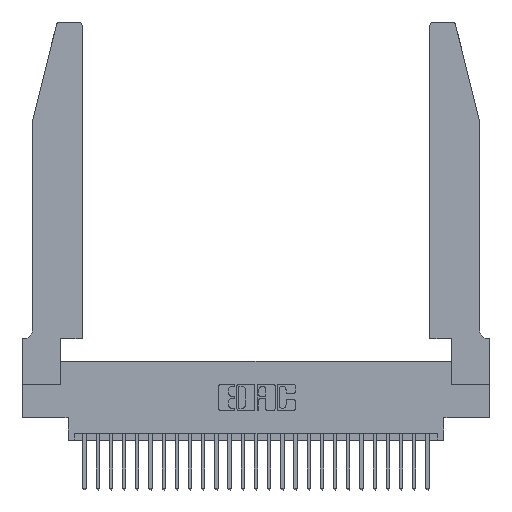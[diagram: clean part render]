
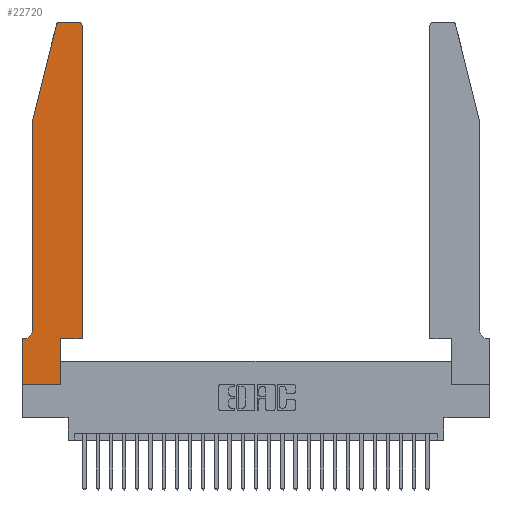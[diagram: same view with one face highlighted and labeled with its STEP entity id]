
A CAD part, top view. The second image highlights one B-rep face of the part: STEP entity #22720.
In plain terms, the highlighted planar face has unit normal (0, 0, 1).
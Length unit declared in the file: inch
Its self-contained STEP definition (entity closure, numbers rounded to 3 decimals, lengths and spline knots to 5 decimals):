
#254 = VERTEX_POINT ( 'NONE', #19557 ) ;
#407 = EDGE_CURVE ( 'NONE', #25255, #20620, #20822, .T. ) ;
#1714 = EDGE_CURVE ( 'NONE', #3235, #7491, #9047, .T. ) ;
#2442 = AXIS2_PLACEMENT_3D ( 'NONE', #22260, #9451, #24450 ) ;
#2991 = CARTESIAN_POINT ( 'NONE',  ( 0.4205, 2.72, 0.37 ) ) ;
#3069 = ORIENTED_EDGE ( 'NONE', *, *, #3690, .T. ) ;
#3218 = ORIENTED_EDGE ( 'NONE', *, *, #407, .T. ) ;
#3228 = DIRECTION ( 'NONE',  ( 0., 1., 0. ) ) ;
#3235 = VERTEX_POINT ( 'NONE', #10721 ) ;
#3276 = VERTEX_POINT ( 'NONE', #25834 ) ;
#3369 = DIRECTION ( 'NONE',  ( -1., 0., 0. ) ) ;
#3472 = DIRECTION ( 'NONE',  ( 0., 0., -1. ) ) ;
#3539 = DIRECTION ( 'NONE',  ( 0., 1., 0. ) ) ;
#3690 = EDGE_CURVE ( 'NONE', #3276, #25255, #16684, .T. ) ;
#3714 = ORIENTED_EDGE ( 'NONE', *, *, #25253, .T. ) ;
#4556 = LINE ( 'NONE', #4732, #15393 ) ;
#4732 = CARTESIAN_POINT ( 'NONE',  ( 0.0755, 2., 0.37 ) ) ;
#4796 = LINE ( 'NONE', #8693, #11289 ) ;
#5183 = CARTESIAN_POINT ( 'NONE',  ( 0., 0.35, 0.37 ) ) ;
#5237 = DIRECTION ( 'NONE',  ( 0., 0., 1. ) ) ;
#5478 = VECTOR ( 'NONE', #22611, 39.37008 ) ;
#5980 = VECTOR ( 'NONE', #3539, 39.37008 ) ;
#6253 = ORIENTED_EDGE ( 'NONE', *, *, #11063, .T. ) ;
#6479 = EDGE_CURVE ( 'NONE', #15203, #18453, #12311, .T. ) ;
#6939 = DIRECTION ( 'NONE',  ( 0., -1., 0. ) ) ;
#6969 = CARTESIAN_POINT ( 'NONE',  ( 0.284, 2.75, 0.37 ) ) ;
#7439 = ORIENTED_EDGE ( 'NONE', *, *, #18773, .T. ) ;
#7491 = VERTEX_POINT ( 'NONE', #19659 ) ;
#7611 = DIRECTION ( 'NONE',  ( 1., 0., 0. ) ) ;
#7701 = DIRECTION ( 'NONE',  ( 0., 0., 1. ) ) ;
#8693 = CARTESIAN_POINT ( 'NONE',  ( 0., 0., 0.37 ) ) ;
#8713 = EDGE_CURVE ( 'NONE', #15310, #26716, #26998, .T. ) ;
#8906 = ORIENTED_EDGE ( 'NONE', *, *, #16973, .T. ) ;
#9047 = LINE ( 'NONE', #19254, #19760 ) ;
#9451 = DIRECTION ( 'NONE',  ( 0., 0., 1. ) ) ;
#9838 = VECTOR ( 'NONE', #25774, 39.37008 ) ;
#10054 = CARTESIAN_POINT ( 'NONE',  ( 0.2865, 0.35, 0.37 ) ) ;
#10562 = VERTEX_POINT ( 'NONE', #25782 ) ;
#10721 = CARTESIAN_POINT ( 'NONE',  ( 0., 0., 0.37 ) ) ;
#10998 = VECTOR ( 'NONE', #3228, 39.37008 ) ;
#11063 = EDGE_CURVE ( 'NONE', #10562, #15203, #26892, .T. ) ;
#11289 = VECTOR ( 'NONE', #25888, 39.37008 ) ;
#11610 = CARTESIAN_POINT ( 'NONE',  ( 0.4505, 2.72, 0.37 ) ) ;
#11752 = LINE ( 'NONE', #10054, #5980 ) ;
#12311 = LINE ( 'NONE', #24909, #24390 ) ;
#12531 = EDGE_CURVE ( 'NONE', #18453, #3235, #4796, .T. ) ;
#13616 = ORIENTED_EDGE ( 'NONE', *, *, #17821, .T. ) ;
#14509 = FACE_OUTER_BOUND ( 'NONE', #27955, .T. ) ;
#15203 = VERTEX_POINT ( 'NONE', #18463 ) ;
#15310 = VERTEX_POINT ( 'NONE', #28075 ) ;
#15393 = VECTOR ( 'NONE', #6939, 39.37008 ) ;
#15480 = DIRECTION ( 'NONE',  ( 1., 0., 0. ) ) ;
#16153 = CARTESIAN_POINT ( 'NONE',  ( 0.2605, 2.75, 0.37 ) ) ;
#16378 = ORIENTED_EDGE ( 'NONE', *, *, #12531, .T. ) ;
#16444 = CARTESIAN_POINT ( 'NONE',  ( 0.0055, 0.42, 0.37 ) ) ;
#16574 = AXIS2_PLACEMENT_3D ( 'NONE', #18182, #5237, #20313 ) ;
#16684 = LINE ( 'NONE', #26951, #10998 ) ;
#16885 = ORIENTED_EDGE ( 'NONE', *, *, #1714, .T. ) ;
#16973 = EDGE_CURVE ( 'NONE', #7491, #254, #11752, .T. ) ;
#17649 = LINE ( 'NONE', #16153, #5478 ) ;
#17795 = ORIENTED_EDGE ( 'NONE', *, *, #19854, .T. ) ;
#17821 = EDGE_CURVE ( 'NONE', #26716, #10562, #4556, .T. ) ;
#18088 = PLANE ( 'NONE',  #16574 ) ;
#18182 = CARTESIAN_POINT ( 'NONE',  ( 0., 0.35, 0.37 ) ) ;
#18453 = VERTEX_POINT ( 'NONE', #5183 ) ;
#18463 = CARTESIAN_POINT ( 'NONE',  ( 0.0055, 0.35, 0.37 ) ) ;
#18616 = DIRECTION ( 'NONE',  ( -1., 0., 0. ) ) ;
#18773 = EDGE_CURVE ( 'NONE', #254, #3276, #26810, .T. ) ;
#19254 = CARTESIAN_POINT ( 'NONE',  ( 0., 0., 0.37 ) ) ;
#19557 = CARTESIAN_POINT ( 'NONE',  ( 0.2865, 0.35, 0.37 ) ) ;
#19659 = CARTESIAN_POINT ( 'NONE',  ( 0.2865, 0., 0.37 ) ) ;
#19760 = VECTOR ( 'NONE', #15480, 39.37008 ) ;
#19854 = EDGE_CURVE ( 'NONE', #20620, #24449, #17649, .T. ) ;
#19909 = ORIENTED_EDGE ( 'NONE', *, *, #8713, .T. ) ;
#20313 = DIRECTION ( 'NONE',  ( 1., 0., 0. ) ) ;
#20620 = VERTEX_POINT ( 'NONE', #23418 ) ;
#20822 = CIRCLE ( 'NONE', #25038, 0.03 ) ;
#21037 = VECTOR ( 'NONE', #25468, 39.37008 ) ;
#22260 = CARTESIAN_POINT ( 'NONE',  ( 0.284, 2.72, 0.37 ) ) ;
#22273 = AXIS2_PLACEMENT_3D ( 'NONE', #16444, #3472, #18616 ) ;
#22611 = DIRECTION ( 'NONE',  ( -1., 0., 0. ) ) ;
#22720 = ADVANCED_FACE ( 'NONE', ( #14509 ), #18088, .T. ) ;
#22764 = CIRCLE ( 'NONE', #2442, 0.03 ) ;
#23418 = CARTESIAN_POINT ( 'NONE',  ( 0.4205, 2.75, 0.37 ) ) ;
#23565 = CARTESIAN_POINT ( 'NONE',  ( 0.0755, 2., 0.37 ) ) ;
#24064 = ORIENTED_EDGE ( 'NONE', *, *, #6479, .T. ) ;
#24390 = VECTOR ( 'NONE', #3369, 39.37008 ) ;
#24449 = VERTEX_POINT ( 'NONE', #6969 ) ;
#24450 = DIRECTION ( 'NONE',  ( 1., 0., 0. ) ) ;
#24765 = CARTESIAN_POINT ( 'NONE',  ( 0.0755, 2., 0.37 ) ) ;
#24909 = CARTESIAN_POINT ( 'NONE',  ( 0.0755, 0.35, 0.37 ) ) ;
#25038 = AXIS2_PLACEMENT_3D ( 'NONE', #2991, #7701, #7611 ) ;
#25253 = EDGE_CURVE ( 'NONE', #24449, #15310, #22764, .T. ) ;
#25255 = VERTEX_POINT ( 'NONE', #11610 ) ;
#25468 = DIRECTION ( 'NONE',  ( 1., 0., 0. ) ) ;
#25774 = DIRECTION ( 'NONE',  ( -0.239, -0.971, 0. ) ) ;
#25782 = CARTESIAN_POINT ( 'NONE',  ( 0.0755, 0.42, 0.37 ) ) ;
#25834 = CARTESIAN_POINT ( 'NONE',  ( 0.4505, 0.35, 0.37 ) ) ;
#25888 = DIRECTION ( 'NONE',  ( 0., -1., 0. ) ) ;
#26716 = VERTEX_POINT ( 'NONE', #24765 ) ;
#26810 = LINE ( 'NONE', #27641, #21037 ) ;
#26892 = CIRCLE ( 'NONE', #22273, 0.07 ) ;
#26951 = CARTESIAN_POINT ( 'NONE',  ( 0.4505, 0.35, 0.37 ) ) ;
#26998 = LINE ( 'NONE', #23565, #9838 ) ;
#27641 = CARTESIAN_POINT ( 'NONE',  ( 0.4505, 0.35, 0.37 ) ) ;
#27955 = EDGE_LOOP ( 'NONE', ( #17795, #3714, #19909, #13616, #6253, #24064, #16378, #16885, #8906, #7439, #3069, #3218 ) ) ;
#28075 = CARTESIAN_POINT ( 'NONE',  ( 0.25487, 2.72718, 0.37 ) ) ;
